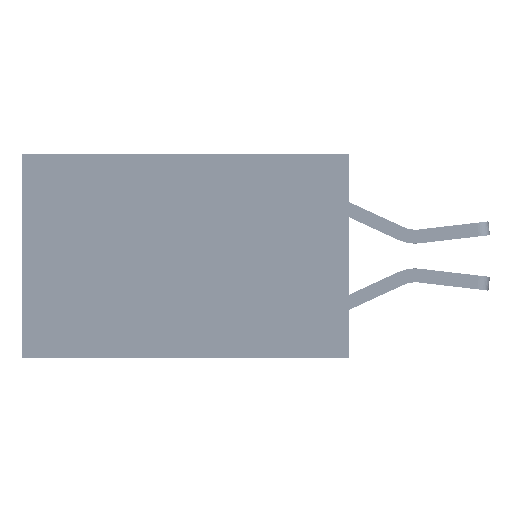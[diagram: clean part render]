
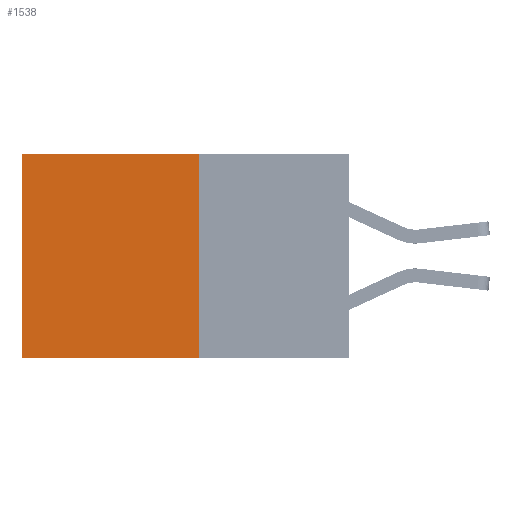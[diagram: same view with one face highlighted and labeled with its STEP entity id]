
A CAD part, left-side view. The second image highlights one B-rep face of the part: STEP entity #1538.
In plain terms, the highlighted planar face has unit normal (-1, 0, 0).
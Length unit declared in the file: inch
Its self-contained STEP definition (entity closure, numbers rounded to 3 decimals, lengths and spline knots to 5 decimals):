
#695 = DIRECTION ( 'NONE',  ( 0., 0., -1. ) ) ;
#759 = VECTOR ( 'NONE', #24962, 39.37008 ) ;
#1273 = ORIENTED_EDGE ( 'NONE', *, *, #10342, .F. ) ;
#1538 = ADVANCED_FACE ( 'NONE', ( #11148 ), #26800, .F. ) ;
#1615 = VECTOR ( 'NONE', #31219, 39.37008 ) ;
#2199 = EDGE_LOOP ( 'NONE', ( #17755, #1273, #32142, #14690 ) ) ;
#2546 = VECTOR ( 'NONE', #11360, 39.37008 ) ;
#3620 = EDGE_CURVE ( 'NONE', #21196, #14814, #7980, .T. ) ;
#5397 = EDGE_CURVE ( 'NONE', #21196, #34526, #16102, .T. ) ;
#6603 = VECTOR ( 'NONE', #695, 39.37008 ) ;
#7980 = LINE ( 'NONE', #25013, #759 ) ;
#10342 = EDGE_CURVE ( 'NONE', #34526, #31346, #24281, .T. ) ;
#10983 = CARTESIAN_POINT ( 'NONE',  ( 0.277, 0.27, -0.37 ) ) ;
#11148 = FACE_OUTER_BOUND ( 'NONE', #2199, .T. ) ;
#11360 = DIRECTION ( 'NONE',  ( 0., 1., 0. ) ) ;
#13731 = CARTESIAN_POINT ( 'NONE',  ( 0.277, 0.27, -0.37 ) ) ;
#14690 = ORIENTED_EDGE ( 'NONE', *, *, #3620, .T. ) ;
#14814 = VERTEX_POINT ( 'NONE', #32012 ) ;
#14979 = CARTESIAN_POINT ( 'NONE',  ( 0.277, 0.59, -0.37 ) ) ;
#15911 = EDGE_CURVE ( 'NONE', #14814, #31346, #21085, .T. ) ;
#16102 = LINE ( 'NONE', #32113, #1615 ) ;
#16803 = AXIS2_PLACEMENT_3D ( 'NONE', #28861, #17912, #23087 ) ;
#17755 = ORIENTED_EDGE ( 'NONE', *, *, #15911, .T. ) ;
#17912 = DIRECTION ( 'NONE',  ( 1., 0., 0. ) ) ;
#21085 = LINE ( 'NONE', #33198, #6603 ) ;
#21196 = VERTEX_POINT ( 'NONE', #25883 ) ;
#23087 = DIRECTION ( 'NONE',  ( 0., 0., -1. ) ) ;
#24281 = LINE ( 'NONE', #10983, #2546 ) ;
#24962 = DIRECTION ( 'NONE',  ( 0., 1., 0. ) ) ;
#25013 = CARTESIAN_POINT ( 'NONE',  ( 0.277, 0.27, 0. ) ) ;
#25883 = CARTESIAN_POINT ( 'NONE',  ( 0.277, 0.27, 0. ) ) ;
#26800 = PLANE ( 'NONE',  #16803 ) ;
#28861 = CARTESIAN_POINT ( 'NONE',  ( 0.277, 0.27, -0.37 ) ) ;
#31219 = DIRECTION ( 'NONE',  ( 0., 0., -1. ) ) ;
#31346 = VERTEX_POINT ( 'NONE', #14979 ) ;
#32012 = CARTESIAN_POINT ( 'NONE',  ( 0.277, 0.59, 0. ) ) ;
#32113 = CARTESIAN_POINT ( 'NONE',  ( 0.277, 0.27, -0.37 ) ) ;
#32142 = ORIENTED_EDGE ( 'NONE', *, *, #5397, .F. ) ;
#33198 = CARTESIAN_POINT ( 'NONE',  ( 0.277, 0.59, -0.37 ) ) ;
#34526 = VERTEX_POINT ( 'NONE', #13731 ) ;
